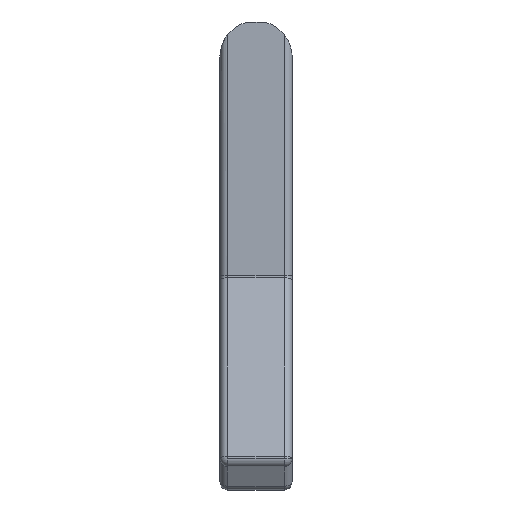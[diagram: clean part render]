
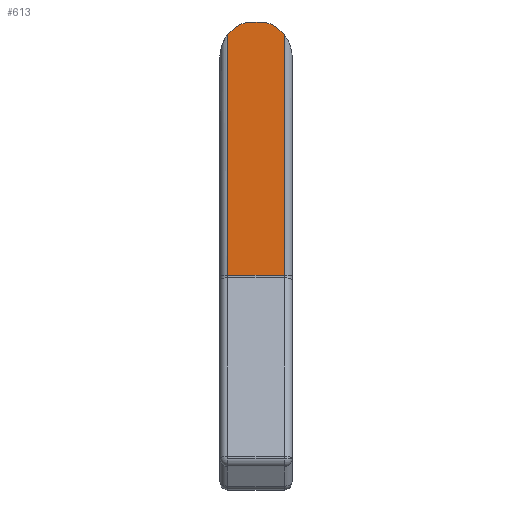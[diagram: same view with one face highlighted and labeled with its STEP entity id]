
A CAD part, top view. The second image highlights one B-rep face of the part: STEP entity #613.
In plain terms, the highlighted planar face has unit normal (0, 0, 1).
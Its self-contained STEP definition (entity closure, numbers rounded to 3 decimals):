
#15 = VERTEX_POINT ( 'NONE', #831 ) ;
#25 = VERTEX_POINT ( 'NONE', #835 ) ;
#30 = VERTEX_POINT ( 'NONE', #959 ) ;
#33 = VERTEX_POINT ( 'NONE', #956 ) ;
#38 = VERTEX_POINT ( 'NONE', #951 ) ;
#45 = VERTEX_POINT ( 'NONE', #945 ) ;
#613 = ADVANCED_FACE ( 'NONE', ( #2728 ), #3048, .F. ) ;
#730 = ORIENTED_EDGE ( 'NONE', *, *, #2685, .T. ) ;
#731 = ORIENTED_EDGE ( 'NONE', *, *, #2651, .T. ) ;
#732 = ORIENTED_EDGE ( 'NONE', *, *, #2795, .F. ) ;
#733 = ORIENTED_EDGE ( 'NONE', *, *, #2778, .T. ) ;
#734 = ORIENTED_EDGE ( 'NONE', *, *, #2796, .T. ) ;
#736 = ORIENTED_EDGE ( 'NONE', *, *, #2798, .F. ) ;
#831 = CARTESIAN_POINT ( 'NONE',  ( 5.559, 43.374, 0. ) ) ;
#835 = CARTESIAN_POINT ( 'NONE',  ( 8., 41.828, 0. ) ) ;
#945 = CARTESIAN_POINT ( 'NONE',  ( 1., 11.76, 0. ) ) ;
#951 = CARTESIAN_POINT ( 'NONE',  ( 8., 11.76, 0. ) ) ;
#956 = CARTESIAN_POINT ( 'NONE',  ( 1., 41.828, 0. ) ) ;
#959 = CARTESIAN_POINT ( 'NONE',  ( 3.441, 43.374, 0. ) ) ;
#1090 = AXIS2_PLACEMENT_3D ( 'NONE', #3038, #3045, #3044 ) ;
#1300 = LINE ( 'NONE', #3198, #1302 ) ;
#1302 = VECTOR ( 'NONE', #3197, 1000. ) ;
#1345 = LINE ( 'NONE', #3388, #1350 ) ;
#1350 = VECTOR ( 'NONE', #3389, 1000. ) ;
#1394 = LINE ( 'NONE', #3494, #1396 ) ;
#1396 = VECTOR ( 'NONE', #3495, 1000. ) ;
#1414 = LINE ( 'NONE', #3542, #1419 ) ;
#1417 = CIRCLE ( 'NONE', #2830, 4.5 ) ;
#1419 = VECTOR ( 'NONE', #3549, 1000. ) ;
#1420 = CIRCLE ( 'NONE', #2831, 4.5 ) ;
#2418 = EDGE_LOOP ( 'NONE', ( #736, #734, #732, #733, #731, #730 ) ) ;
#2651 = EDGE_CURVE ( 'NONE', #45, #38, #1300, .T. ) ;
#2685 = EDGE_CURVE ( 'NONE', #38, #25, #1345, .T. ) ;
#2728 = FACE_OUTER_BOUND ( 'NONE', #2418, .T. ) ;
#2778 = EDGE_CURVE ( 'NONE', #33, #45, #1394, .T. ) ;
#2795 = EDGE_CURVE ( 'NONE', #33, #30, #1417, .T. ) ;
#2796 = EDGE_CURVE ( 'NONE', #15, #30, #1414, .T. ) ;
#2798 = EDGE_CURVE ( 'NONE', #15, #25, #1420, .T. ) ;
#2830 = AXIS2_PLACEMENT_3D ( 'NONE', #3557, #3558, #3559 ) ;
#2831 = AXIS2_PLACEMENT_3D ( 'NONE', #3563, #3564, #3565 ) ;
#3038 = CARTESIAN_POINT ( 'NONE',  ( 9., 0., 0. ) ) ;
#3044 = DIRECTION ( 'NONE',  ( -1., 0., 0. ) ) ;
#3045 = DIRECTION ( 'NONE',  ( 0., 0., -1. ) ) ;
#3048 = PLANE ( 'NONE',  #1090 ) ;
#3197 = DIRECTION ( 'NONE',  ( 1., 0., 0. ) ) ;
#3198 = CARTESIAN_POINT ( 'NONE',  ( 9., 11.76, 0. ) ) ;
#3388 = CARTESIAN_POINT ( 'NONE',  ( 8., 0., 0. ) ) ;
#3389 = DIRECTION ( 'NONE',  ( 0., 1., 0. ) ) ;
#3494 = CARTESIAN_POINT ( 'NONE',  ( 1., 11.76, 0. ) ) ;
#3495 = DIRECTION ( 'NONE',  ( 0., -1., 0. ) ) ;
#3542 = CARTESIAN_POINT ( 'NONE',  ( 9., 43.374, 0. ) ) ;
#3549 = DIRECTION ( 'NONE',  ( -1., 0., 0. ) ) ;
#3557 = CARTESIAN_POINT ( 'NONE',  ( 4.5, 39., 0. ) ) ;
#3558 = DIRECTION ( 'NONE',  ( 0., 0., -1. ) ) ;
#3559 = DIRECTION ( 'NONE',  ( -1., 0., 0. ) ) ;
#3563 = CARTESIAN_POINT ( 'NONE',  ( 4.5, 39., 0. ) ) ;
#3564 = DIRECTION ( 'NONE',  ( 0., 0., -1. ) ) ;
#3565 = DIRECTION ( 'NONE',  ( -1., 0., 0. ) ) ;
